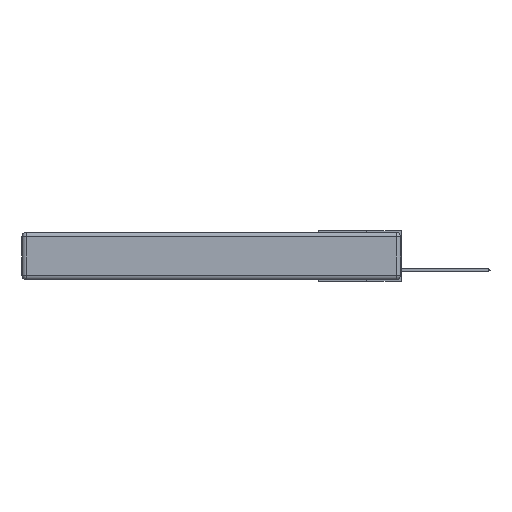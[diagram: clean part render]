
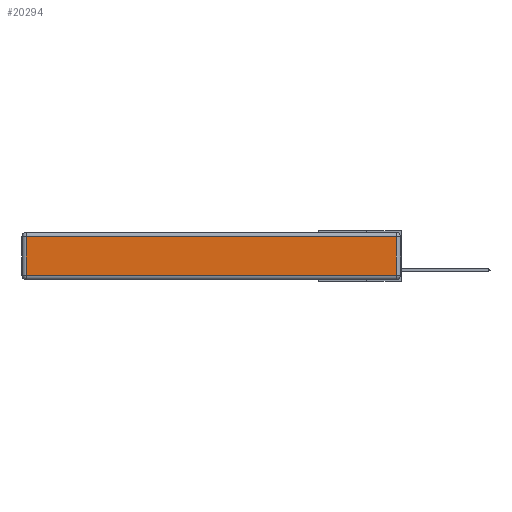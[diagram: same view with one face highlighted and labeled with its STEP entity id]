
A CAD part, left-side view. The second image highlights one B-rep face of the part: STEP entity #20294.
In plain terms, the highlighted planar face has unit normal (-1, 0, 0).
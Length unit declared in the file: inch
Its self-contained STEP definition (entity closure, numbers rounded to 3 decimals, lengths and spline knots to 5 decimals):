
#64 = LINE ( 'NONE', #10183, #5497 ) ;
#537 = VERTEX_POINT ( 'NONE', #16690 ) ;
#619 = LINE ( 'NONE', #14709, #10728 ) ;
#2275 = CARTESIAN_POINT ( 'NONE',  ( 0., 0.03, -0.313 ) ) ;
#2623 = DIRECTION ( 'NONE',  ( -1., 0., 0. ) ) ;
#2730 = CARTESIAN_POINT ( 'NONE',  ( 0., 2.72, -0.343 ) ) ;
#2813 = ORIENTED_EDGE ( 'NONE', *, *, #3789, .T. ) ;
#3132 = CARTESIAN_POINT ( 'NONE',  ( 0., 2.75, -0.03 ) ) ;
#3789 = EDGE_CURVE ( 'NONE', #15646, #537, #619, .T. ) ;
#4141 = ORIENTED_EDGE ( 'NONE', *, *, #11045, .T. ) ;
#5284 = DIRECTION ( 'NONE',  ( 0., -1., 0. ) ) ;
#5497 = VECTOR ( 'NONE', #5284, 39.37008 ) ;
#5573 = LINE ( 'NONE', #3132, #17214 ) ;
#7394 = DIRECTION ( 'NONE',  ( 0., 1., 0. ) ) ;
#7943 = ORIENTED_EDGE ( 'NONE', *, *, #18632, .T. ) ;
#7959 = VERTEX_POINT ( 'NONE', #10444 ) ;
#8709 = VERTEX_POINT ( 'NONE', #14622 ) ;
#10183 = CARTESIAN_POINT ( 'NONE',  ( 0., 0., -0.313 ) ) ;
#10444 = CARTESIAN_POINT ( 'NONE',  ( 0., 2.72, -0.03 ) ) ;
#10728 = VECTOR ( 'NONE', #16113, 39.37008 ) ;
#11045 = EDGE_CURVE ( 'NONE', #537, #7959, #5573, .T. ) ;
#13171 = LINE ( 'NONE', #2730, #13668 ) ;
#13668 = VECTOR ( 'NONE', #20006, 39.37008 ) ;
#14622 = CARTESIAN_POINT ( 'NONE',  ( 0., 2.72, -0.313 ) ) ;
#14709 = CARTESIAN_POINT ( 'NONE',  ( 0., 0.03, -0.343 ) ) ;
#15165 = DIRECTION ( 'NONE',  ( 0., 0., 1. ) ) ;
#15646 = VERTEX_POINT ( 'NONE', #2275 ) ;
#16097 = AXIS2_PLACEMENT_3D ( 'NONE', #16990, #2623, #15165 ) ;
#16113 = DIRECTION ( 'NONE',  ( 0., 0., 1. ) ) ;
#16443 = ORIENTED_EDGE ( 'NONE', *, *, #20435, .T. ) ;
#16690 = CARTESIAN_POINT ( 'NONE',  ( 0., 0.03, -0.03 ) ) ;
#16990 = CARTESIAN_POINT ( 'NONE',  ( 0., 0., -0.343 ) ) ;
#17214 = VECTOR ( 'NONE', #7394, 39.37008 ) ;
#18632 = EDGE_CURVE ( 'NONE', #7959, #8709, #13171, .T. ) ;
#18666 = PLANE ( 'NONE',  #16097 ) ;
#19286 = EDGE_LOOP ( 'NONE', ( #16443, #2813, #4141, #7943 ) ) ;
#20006 = DIRECTION ( 'NONE',  ( 0., 0., -1. ) ) ;
#20113 = FACE_OUTER_BOUND ( 'NONE', #19286, .T. ) ;
#20294 = ADVANCED_FACE ( 'NONE', ( #20113 ), #18666, .T. ) ;
#20435 = EDGE_CURVE ( 'NONE', #8709, #15646, #64, .T. ) ;
